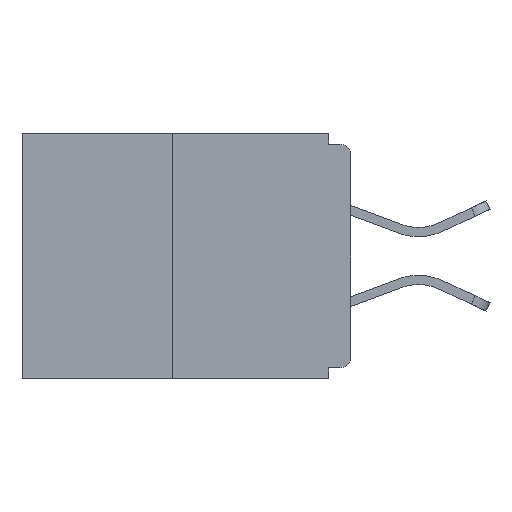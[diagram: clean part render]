
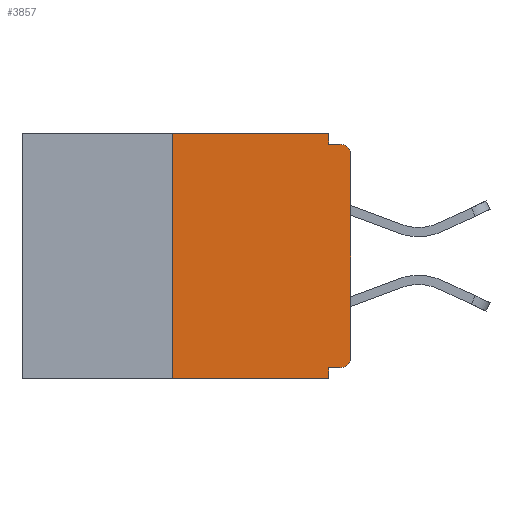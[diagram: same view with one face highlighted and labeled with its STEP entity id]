
A CAD part, left-side view. The second image highlights one B-rep face of the part: STEP entity #3857.
In plain terms, the highlighted planar face has unit normal (-1, 0, 0).
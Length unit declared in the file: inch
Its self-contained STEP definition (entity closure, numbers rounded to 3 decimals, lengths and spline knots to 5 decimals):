
#284 = DIRECTION ( 'NONE',  ( 0., 0., -1. ) ) ;
#1113 = EDGE_CURVE ( 'NONE', #8282, #7370, #3108, .T. ) ;
#1141 = LINE ( 'NONE', #6457, #3062 ) ;
#1198 = ORIENTED_EDGE ( 'NONE', *, *, #12587, .F. ) ;
#1241 = VECTOR ( 'NONE', #19518, 39.37008 ) ;
#1331 = CARTESIAN_POINT ( 'NONE',  ( 0., 0., -0.03 ) ) ;
#1838 = FACE_OUTER_BOUND ( 'NONE', #11365, .T. ) ;
#1911 = VECTOR ( 'NONE', #4270, 39.37008 ) ;
#2020 = VERTEX_POINT ( 'NONE', #12638 ) ;
#2324 = CARTESIAN_POINT ( 'NONE',  ( 0., 0., -0.313 ) ) ;
#2481 = DIRECTION ( 'NONE',  ( 0., 0., -1. ) ) ;
#2535 = DIRECTION ( 'NONE',  ( 0., 0., -1. ) ) ;
#2623 = CARTESIAN_POINT ( 'NONE',  ( 0., 0.25, -0.343 ) ) ;
#3062 = VECTOR ( 'NONE', #15995, 39.37008 ) ;
#3108 = LINE ( 'NONE', #10453, #8240 ) ;
#3133 = EDGE_CURVE ( 'NONE', #2020, #3542, #1141, .T. ) ;
#3542 = VERTEX_POINT ( 'NONE', #10132 ) ;
#3761 = LINE ( 'NONE', #5446, #19828 ) ;
#3857 = ADVANCED_FACE ( 'NONE', ( #1838 ), #20144, .F. ) ;
#3886 = CARTESIAN_POINT ( 'NONE',  ( 0., 0.031, -0.328 ) ) ;
#4072 = EDGE_CURVE ( 'NONE', #8282, #9819, #3761, .T. ) ;
#4122 = CARTESIAN_POINT ( 'NONE',  ( 0., 0.031, 0. ) ) ;
#4128 = LINE ( 'NONE', #10373, #15391 ) ;
#4214 = VERTEX_POINT ( 'NONE', #18041 ) ;
#4270 = DIRECTION ( 'NONE',  ( 0., -1., 0. ) ) ;
#4626 = CARTESIAN_POINT ( 'NONE',  ( 0., 0.46, 0. ) ) ;
#4691 = DIRECTION ( 'NONE',  ( 1., 0., 0. ) ) ;
#4819 = ORIENTED_EDGE ( 'NONE', *, *, #9929, .T. ) ;
#5446 = CARTESIAN_POINT ( 'NONE',  ( 0., 0.46, -0.343 ) ) ;
#5486 = VECTOR ( 'NONE', #284, 39.37008 ) ;
#5492 = CARTESIAN_POINT ( 'NONE',  ( 0., 0.015, -0.313 ) ) ;
#5610 = LINE ( 'NONE', #13066, #1241 ) ;
#5743 = ORIENTED_EDGE ( 'NONE', *, *, #1113, .F. ) ;
#5773 = DIRECTION ( 'NONE',  ( 0., 0., -1. ) ) ;
#5822 = ORIENTED_EDGE ( 'NONE', *, *, #3133, .F. ) ;
#5941 = CIRCLE ( 'NONE', #6991, 0.015 ) ;
#6457 = CARTESIAN_POINT ( 'NONE',  ( 0., 0., -0.015 ) ) ;
#6991 = AXIS2_PLACEMENT_3D ( 'NONE', #5492, #17960, #2481 ) ;
#7180 = VERTEX_POINT ( 'NONE', #2324 ) ;
#7370 = VERTEX_POINT ( 'NONE', #19907 ) ;
#7475 = CIRCLE ( 'NONE', #17818, 0.015 ) ;
#7526 = ORIENTED_EDGE ( 'NONE', *, *, #11675, .F. ) ;
#7875 = ORIENTED_EDGE ( 'NONE', *, *, #4072, .T. ) ;
#8191 = EDGE_CURVE ( 'NONE', #7180, #17428, #5610, .T. ) ;
#8240 = VECTOR ( 'NONE', #16757, 39.37008 ) ;
#8282 = VERTEX_POINT ( 'NONE', #2623 ) ;
#8361 = DIRECTION ( 'NONE',  ( 0., 1., 0. ) ) ;
#9817 = VERTEX_POINT ( 'NONE', #3886 ) ;
#9819 = VERTEX_POINT ( 'NONE', #9946 ) ;
#9929 = EDGE_CURVE ( 'NONE', #17428, #3542, #7475, .T. ) ;
#9946 = CARTESIAN_POINT ( 'NONE',  ( 0., 0.031, -0.343 ) ) ;
#10132 = CARTESIAN_POINT ( 'NONE',  ( 0., 0.015, -0.015 ) ) ;
#10275 = ORIENTED_EDGE ( 'NONE', *, *, #8191, .T. ) ;
#10373 = CARTESIAN_POINT ( 'NONE',  ( 0., 0., -0.328 ) ) ;
#10453 = CARTESIAN_POINT ( 'NONE',  ( 0., 0.25, 0. ) ) ;
#10476 = EDGE_CURVE ( 'NONE', #15238, #9817, #4128, .T. ) ;
#10683 = EDGE_CURVE ( 'NONE', #7370, #4214, #12869, .T. ) ;
#11365 = EDGE_LOOP ( 'NONE', ( #12163, #5743, #7875, #1198, #13455, #18443, #10275, #4819, #5822, #7526 ) ) ;
#11675 = EDGE_CURVE ( 'NONE', #4214, #2020, #11828, .T. ) ;
#11710 = CARTESIAN_POINT ( 'NONE',  ( 0., 0.015, -0.03 ) ) ;
#11793 = LINE ( 'NONE', #14255, #5486 ) ;
#11828 = LINE ( 'NONE', #4122, #17959 ) ;
#12163 = ORIENTED_EDGE ( 'NONE', *, *, #10683, .F. ) ;
#12230 = CARTESIAN_POINT ( 'NONE',  ( 0., 0.46, 0. ) ) ;
#12234 = EDGE_CURVE ( 'NONE', #15238, #7180, #5941, .T. ) ;
#12587 = EDGE_CURVE ( 'NONE', #9817, #9819, #11793, .T. ) ;
#12638 = CARTESIAN_POINT ( 'NONE',  ( 0., 0.031, -0.015 ) ) ;
#12869 = LINE ( 'NONE', #12230, #1911 ) ;
#13066 = CARTESIAN_POINT ( 'NONE',  ( 0., 0., 0. ) ) ;
#13455 = ORIENTED_EDGE ( 'NONE', *, *, #10476, .F. ) ;
#14255 = CARTESIAN_POINT ( 'NONE',  ( 0., 0.031, -0.343 ) ) ;
#14794 = DIRECTION ( 'NONE',  ( 0., -1., 0. ) ) ;
#14907 = AXIS2_PLACEMENT_3D ( 'NONE', #4626, #4691, #5773 ) ;
#14953 = DIRECTION ( 'NONE',  ( 0., 0., -1. ) ) ;
#15075 = DIRECTION ( 'NONE',  ( -1., 0., 0. ) ) ;
#15238 = VERTEX_POINT ( 'NONE', #15460 ) ;
#15391 = VECTOR ( 'NONE', #8361, 39.37008 ) ;
#15460 = CARTESIAN_POINT ( 'NONE',  ( 0., 0.015, -0.328 ) ) ;
#15995 = DIRECTION ( 'NONE',  ( 0., -1., 0. ) ) ;
#16757 = DIRECTION ( 'NONE',  ( 0., 0., 1. ) ) ;
#17428 = VERTEX_POINT ( 'NONE', #1331 ) ;
#17818 = AXIS2_PLACEMENT_3D ( 'NONE', #11710, #15075, #2535 ) ;
#17959 = VECTOR ( 'NONE', #14953, 39.37008 ) ;
#17960 = DIRECTION ( 'NONE',  ( -1., 0., 0. ) ) ;
#18041 = CARTESIAN_POINT ( 'NONE',  ( 0., 0.031, 0. ) ) ;
#18443 = ORIENTED_EDGE ( 'NONE', *, *, #12234, .T. ) ;
#19518 = DIRECTION ( 'NONE',  ( 0., 0., 1. ) ) ;
#19828 = VECTOR ( 'NONE', #14794, 39.37008 ) ;
#19907 = CARTESIAN_POINT ( 'NONE',  ( 0., 0.25, 0. ) ) ;
#20144 = PLANE ( 'NONE',  #14907 ) ;
